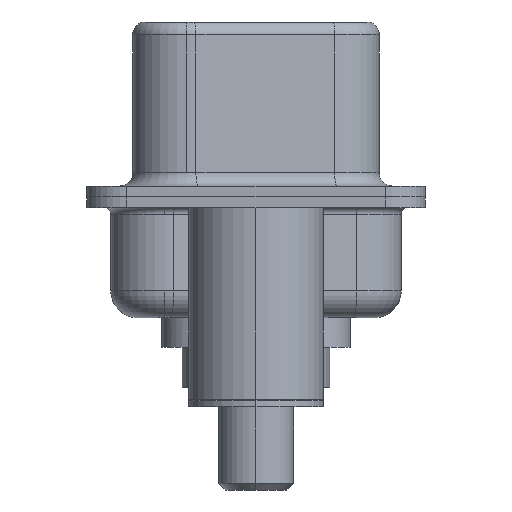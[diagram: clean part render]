
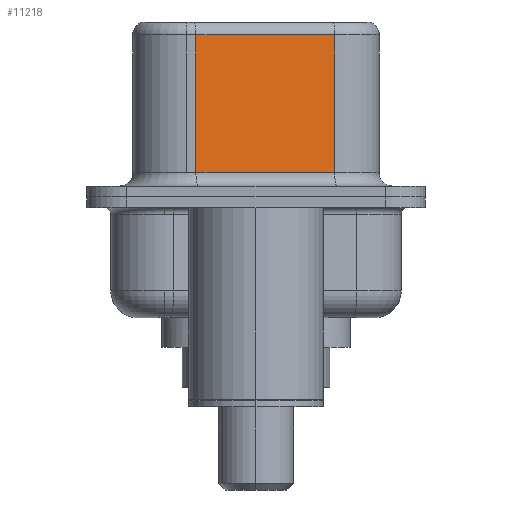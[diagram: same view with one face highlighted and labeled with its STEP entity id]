
A CAD part, left-side view. The second image highlights one B-rep face of the part: STEP entity #11218.
In plain terms, the highlighted planar face has unit normal (-0.985, -0.174, 0).
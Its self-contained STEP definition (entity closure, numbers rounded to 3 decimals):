
#347 = ORIENTED_EDGE ( 'NONE', *, *, #7075, .T. ) ;
#1262 = VERTEX_POINT ( 'NONE', #12460 ) ;
#1478 = LINE ( 'NONE', #2833, #6635 ) ;
#1503 = LINE ( 'NONE', #4536, #3554 ) ;
#2001 = DIRECTION ( 'NONE',  ( -0.174, 0.985, 0. ) ) ;
#2104 = EDGE_CURVE ( 'NONE', #9735, #10859, #2491, .T. ) ;
#2491 = LINE ( 'NONE', #8319, #7690 ) ;
#2833 = CARTESIAN_POINT ( 'NONE',  ( 4.565, -2.927, 6.52 ) ) ;
#2843 = EDGE_LOOP ( 'NONE', ( #10615, #347, #4829, #13090 ) ) ;
#3024 = DIRECTION ( 'NONE',  ( 0.985, 0.174, 0. ) ) ;
#3554 = VECTOR ( 'NONE', #5572, 1000. ) ;
#3807 = AXIS2_PLACEMENT_3D ( 'NONE', #11379, #3024, #10360 ) ;
#4536 = CARTESIAN_POINT ( 'NONE',  ( 3.655, 2.233, 6.52 ) ) ;
#4829 = ORIENTED_EDGE ( 'NONE', *, *, #10170, .T. ) ;
#5572 = DIRECTION ( 'NONE',  ( 0., 0., -1. ) ) ;
#5739 = EDGE_CURVE ( 'NONE', #8981, #10859, #1478, .T. ) ;
#6635 = VECTOR ( 'NONE', #8486, 1000. ) ;
#6831 = CARTESIAN_POINT ( 'NONE',  ( 4.565, -2.927, 6.02 ) ) ;
#7075 = EDGE_CURVE ( 'NONE', #8981, #1262, #11911, .T. ) ;
#7690 = VECTOR ( 'NONE', #9997, 1000. ) ;
#8319 = CARTESIAN_POINT ( 'NONE',  ( 4.565, -2.927, 0.9 ) ) ;
#8486 = DIRECTION ( 'NONE',  ( 0., 0., -1. ) ) ;
#8981 = VERTEX_POINT ( 'NONE', #6831 ) ;
#9268 = CARTESIAN_POINT ( 'NONE',  ( 4.565, -2.927, 6.02 ) ) ;
#9735 = VERTEX_POINT ( 'NONE', #10215 ) ;
#9805 = CARTESIAN_POINT ( 'NONE',  ( 4.565, -2.927, 0.9 ) ) ;
#9997 = DIRECTION ( 'NONE',  ( 0.174, -0.985, 0. ) ) ;
#10170 = EDGE_CURVE ( 'NONE', #1262, #9735, #1503, .T. ) ;
#10215 = CARTESIAN_POINT ( 'NONE',  ( 3.655, 2.233, 0.9 ) ) ;
#10360 = DIRECTION ( 'NONE',  ( -0.174, 0.985, 0. ) ) ;
#10431 = VECTOR ( 'NONE', #2001, 1000. ) ;
#10615 = ORIENTED_EDGE ( 'NONE', *, *, #5739, .F. ) ;
#10859 = VERTEX_POINT ( 'NONE', #9805 ) ;
#11218 = ADVANCED_FACE ( 'NONE', ( #11778 ), #13482, .F. ) ;
#11379 = CARTESIAN_POINT ( 'NONE',  ( 4.565, -2.927, 6.52 ) ) ;
#11778 = FACE_OUTER_BOUND ( 'NONE', #2843, .T. ) ;
#11911 = LINE ( 'NONE', #9268, #10431 ) ;
#12460 = CARTESIAN_POINT ( 'NONE',  ( 3.655, 2.233, 6.02 ) ) ;
#13090 = ORIENTED_EDGE ( 'NONE', *, *, #2104, .T. ) ;
#13482 = PLANE ( 'NONE',  #3807 ) ;
